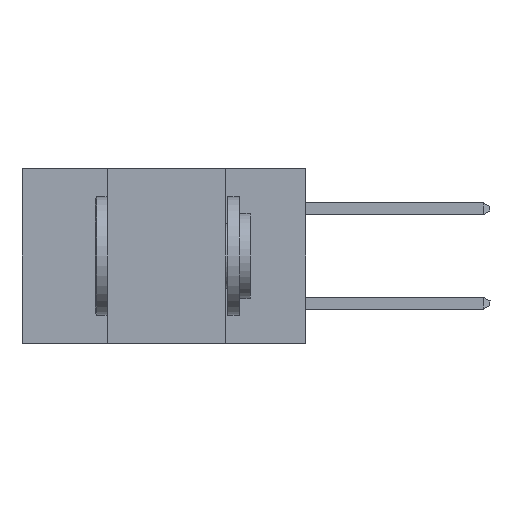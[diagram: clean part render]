
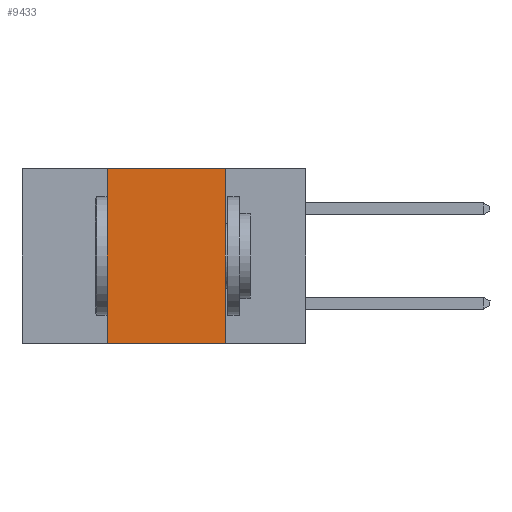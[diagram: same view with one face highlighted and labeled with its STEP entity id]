
A CAD part, left-side view. The second image highlights one B-rep face of the part: STEP entity #9433.
In plain terms, the highlighted planar face has unit normal (-1, 0, 0).
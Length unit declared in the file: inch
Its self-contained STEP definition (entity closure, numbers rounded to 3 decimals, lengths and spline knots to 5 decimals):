
#789 = DIRECTION ( 'NONE',  ( 0., -1., 0. ) ) ;
#875 = CARTESIAN_POINT ( 'NONE',  ( 0., 0.42, 0. ) ) ;
#894 = VERTEX_POINT ( 'NONE', #14181 ) ;
#1902 = DIRECTION ( 'NONE',  ( 1., 0., 0. ) ) ;
#4394 = LINE ( 'NONE', #7406, #13233 ) ;
#6748 = VECTOR ( 'NONE', #14648, 39.37008 ) ;
#7406 = CARTESIAN_POINT ( 'NONE',  ( 0., 0.17, 0. ) ) ;
#9102 = EDGE_LOOP ( 'NONE', ( #10129, #10133, #15221, #20413 ) ) ;
#9433 = ADVANCED_FACE ( 'NONE', ( #14810 ), #20700, .F. ) ;
#10129 = ORIENTED_EDGE ( 'NONE', *, *, #20304, .F. ) ;
#10133 = ORIENTED_EDGE ( 'NONE', *, *, #10782, .F. ) ;
#10242 = VERTEX_POINT ( 'NONE', #20699 ) ;
#10782 = EDGE_CURVE ( 'NONE', #10242, #894, #14709, .T. ) ;
#12165 = CARTESIAN_POINT ( 'NONE',  ( 0., 0.6, -0.37 ) ) ;
#12286 = LINE ( 'NONE', #12165, #6748 ) ;
#12563 = CARTESIAN_POINT ( 'NONE',  ( 0., 0.6, 0. ) ) ;
#12669 = DIRECTION ( 'NONE',  ( 0., 0., -1. ) ) ;
#13233 = VECTOR ( 'NONE', #21883, 39.37008 ) ;
#13384 = CARTESIAN_POINT ( 'NONE',  ( 0., 0.6, 0. ) ) ;
#14181 = CARTESIAN_POINT ( 'NONE',  ( 0., 0.17, 0. ) ) ;
#14648 = DIRECTION ( 'NONE',  ( 0., -1., 0. ) ) ;
#14709 = LINE ( 'NONE', #13384, #16313 ) ;
#14810 = FACE_OUTER_BOUND ( 'NONE', #9102, .T. ) ;
#15221 = ORIENTED_EDGE ( 'NONE', *, *, #18727, .F. ) ;
#15295 = CARTESIAN_POINT ( 'NONE',  ( 0., 0.42, -0.37 ) ) ;
#16313 = VECTOR ( 'NONE', #789, 39.37008 ) ;
#18098 = VERTEX_POINT ( 'NONE', #15295 ) ;
#18439 = CARTESIAN_POINT ( 'NONE',  ( 0., 0.17, -0.37 ) ) ;
#18727 = EDGE_CURVE ( 'NONE', #18098, #10242, #22967, .T. ) ;
#19115 = VECTOR ( 'NONE', #23947, 39.37008 ) ;
#20304 = EDGE_CURVE ( 'NONE', #894, #20432, #4394, .T. ) ;
#20413 = ORIENTED_EDGE ( 'NONE', *, *, #25666, .T. ) ;
#20432 = VERTEX_POINT ( 'NONE', #18439 ) ;
#20699 = CARTESIAN_POINT ( 'NONE',  ( 0., 0.42, 0. ) ) ;
#20700 = PLANE ( 'NONE',  #23793 ) ;
#21883 = DIRECTION ( 'NONE',  ( 0., 0., -1. ) ) ;
#22967 = LINE ( 'NONE', #875, #19115 ) ;
#23793 = AXIS2_PLACEMENT_3D ( 'NONE', #12563, #1902, #12669 ) ;
#23947 = DIRECTION ( 'NONE',  ( 0., 0., 1. ) ) ;
#25666 = EDGE_CURVE ( 'NONE', #18098, #20432, #12286, .T. ) ;
